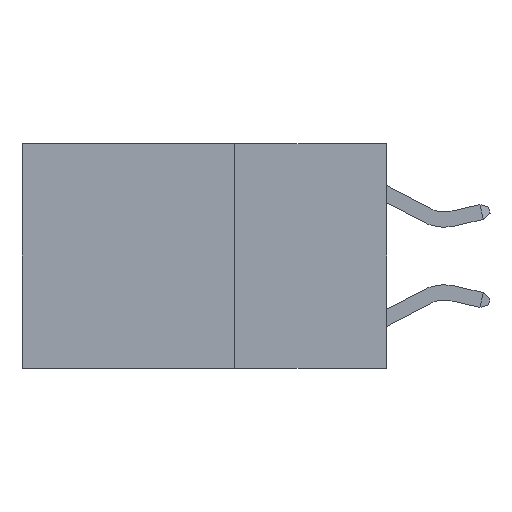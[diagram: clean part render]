
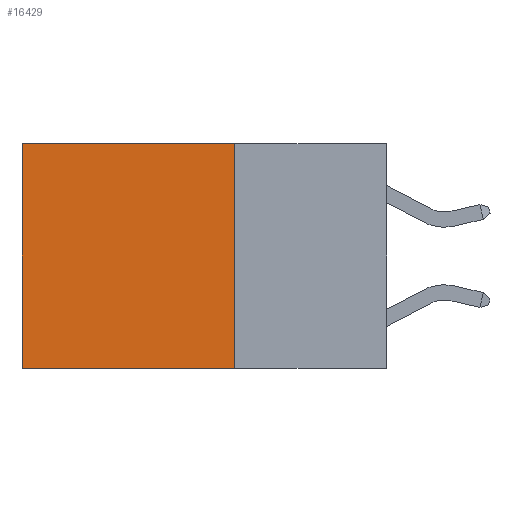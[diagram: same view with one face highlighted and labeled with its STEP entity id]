
A CAD part, left-side view. The second image highlights one B-rep face of the part: STEP entity #16429.
In plain terms, the highlighted planar face has unit normal (-1, 0, 0).
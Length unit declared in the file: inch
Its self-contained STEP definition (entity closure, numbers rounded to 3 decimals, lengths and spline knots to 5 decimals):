
#135 = CARTESIAN_POINT ( 'NONE',  ( 0.2625, 0.6, 0. ) ) ;
#608 = ORIENTED_EDGE ( 'NONE', *, *, #6768, .T. ) ;
#1239 = FACE_OUTER_BOUND ( 'NONE', #14179, .T. ) ;
#1490 = DIRECTION ( 'NONE',  ( 0., 1., 0. ) ) ;
#1592 = DIRECTION ( 'NONE',  ( 0., 0., -1. ) ) ;
#1797 = VECTOR ( 'NONE', #21072, 39.37008 ) ;
#2115 = PLANE ( 'NONE',  #21068 ) ;
#2673 = VERTEX_POINT ( 'NONE', #8199 ) ;
#3156 = VERTEX_POINT ( 'NONE', #12566 ) ;
#4212 = DIRECTION ( 'NONE',  ( 0., 0., -1. ) ) ;
#4280 = VECTOR ( 'NONE', #1592, 39.37008 ) ;
#6720 = VERTEX_POINT ( 'NONE', #22309 ) ;
#6768 = EDGE_CURVE ( 'NONE', #3156, #6720, #10548, .T. ) ;
#7507 = LINE ( 'NONE', #135, #1797 ) ;
#8199 = CARTESIAN_POINT ( 'NONE',  ( 0.2625, 0.6, -0.37 ) ) ;
#8948 = EDGE_CURVE ( 'NONE', #12793, #2673, #19145, .T. ) ;
#9202 = EDGE_CURVE ( 'NONE', #3156, #12793, #20313, .T. ) ;
#9978 = VECTOR ( 'NONE', #11157, 39.37008 ) ;
#10237 = EDGE_CURVE ( 'NONE', #6720, #2673, #7507, .T. ) ;
#10548 = LINE ( 'NONE', #16618, #9978 ) ;
#11121 = CARTESIAN_POINT ( 'NONE',  ( 0.2625, 0.25, 0. ) ) ;
#11157 = DIRECTION ( 'NONE',  ( 0., 1., 0. ) ) ;
#11215 = CARTESIAN_POINT ( 'NONE',  ( 0.2625, 0.25, -0.37 ) ) ;
#12179 = ORIENTED_EDGE ( 'NONE', *, *, #8948, .F. ) ;
#12566 = CARTESIAN_POINT ( 'NONE',  ( 0.2625, 0.25, 0. ) ) ;
#12793 = VERTEX_POINT ( 'NONE', #11215 ) ;
#13628 = DIRECTION ( 'NONE',  ( 1., 0., 0. ) ) ;
#14125 = VECTOR ( 'NONE', #1490, 39.37008 ) ;
#14179 = EDGE_LOOP ( 'NONE', ( #23598, #12179, #17851, #608 ) ) ;
#15770 = CARTESIAN_POINT ( 'NONE',  ( 0.2625, 0.25, 0. ) ) ;
#16363 = CARTESIAN_POINT ( 'NONE',  ( 0.2625, 0.25, -0.37 ) ) ;
#16429 = ADVANCED_FACE ( 'NONE', ( #1239 ), #2115, .F. ) ;
#16618 = CARTESIAN_POINT ( 'NONE',  ( 0.2625, 0.25, 0. ) ) ;
#17851 = ORIENTED_EDGE ( 'NONE', *, *, #9202, .F. ) ;
#19145 = LINE ( 'NONE', #16363, #14125 ) ;
#20313 = LINE ( 'NONE', #11121, #4280 ) ;
#21068 = AXIS2_PLACEMENT_3D ( 'NONE', #15770, #13628, #4212 ) ;
#21072 = DIRECTION ( 'NONE',  ( 0., 0., -1. ) ) ;
#22309 = CARTESIAN_POINT ( 'NONE',  ( 0.2625, 0.6, 0. ) ) ;
#23598 = ORIENTED_EDGE ( 'NONE', *, *, #10237, .T. ) ;
